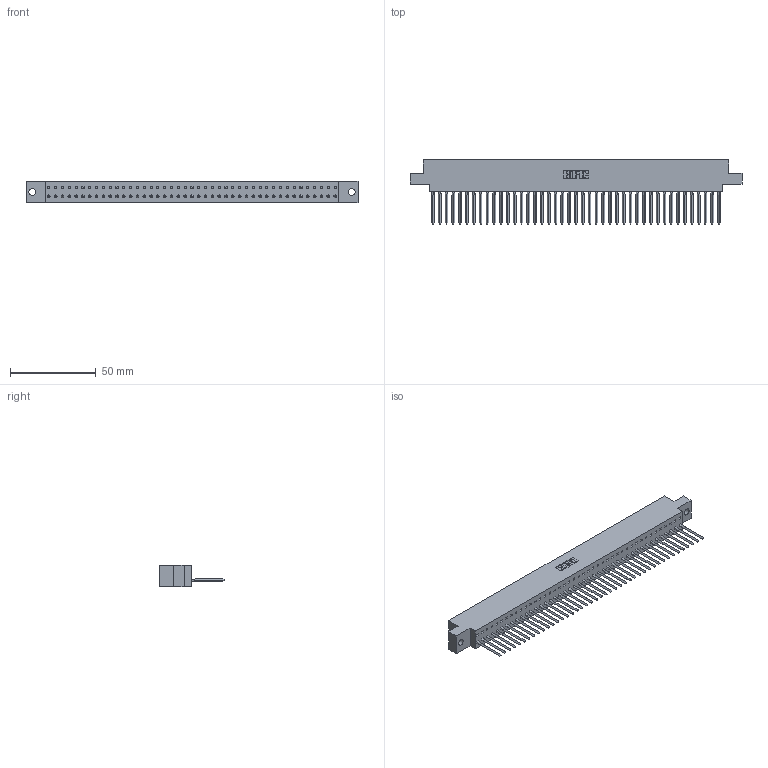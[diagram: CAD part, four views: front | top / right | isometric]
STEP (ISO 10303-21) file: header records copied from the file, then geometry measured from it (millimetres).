
FILE_DESCRIPTION (( 'STEP AP203' ), '1' );
FILE_NAME ('317-043-541-604.STEP', '2020-02-28T01:51:24', ( '' ), ( '' ), 'SwSTEP 2.0', 'SolidWorks 2016', '' );
FILE_SCHEMA (( 'CONFIG_CONTROL_DESIGN' ));
Length unit declared in the file: inch
Products named in the file (3): 317-043-541-604; 317-290-002_541; 317 Part_.156 Dia - TH
Assembly tree (44 placements, depth 2):
  317-043-541-604
    317 Part_.156 Dia - TH
    317-290-002_541  x43
Bounding box: 193.09 x 37.34 x 12.7 mm (x, y, z)
Volume: 31255.7 mm3; surface area: 44017.8 mm2
Topology: 44 solids, 44 shells, 6638 faces, 18937 edges, 12308 vertices
Faces by surface type: plane 5390, cylinder 1076, bspline 172
Entity records: 62192 total; most frequent: CARTESIAN_POINT 11698, ORIENTED_EDGE 10994, DIRECTION 9031, EDGE_CURVE 5497, LINE 5133, VECTOR 5133, VERTEX_POINT 3656, AXIS2_PLACEMENT_3D 1949
